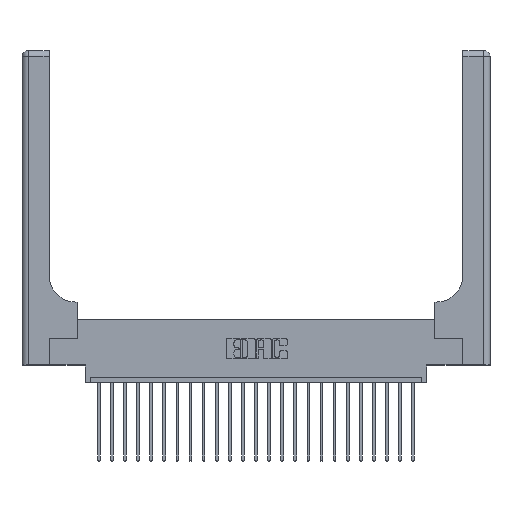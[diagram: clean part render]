
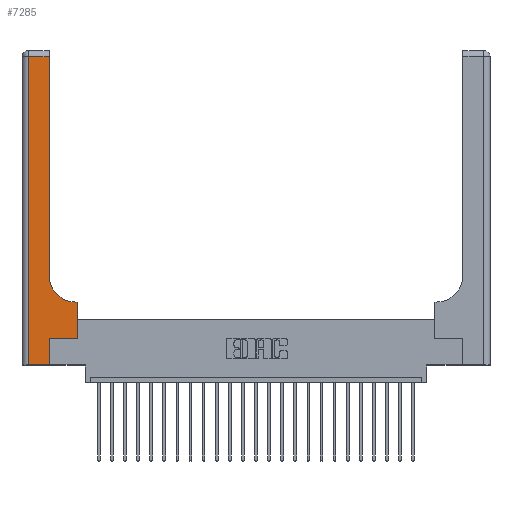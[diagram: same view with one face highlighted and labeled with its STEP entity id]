
A CAD part, top view. The second image highlights one B-rep face of the part: STEP entity #7285.
In plain terms, the highlighted planar face has unit normal (0, 0, 1).
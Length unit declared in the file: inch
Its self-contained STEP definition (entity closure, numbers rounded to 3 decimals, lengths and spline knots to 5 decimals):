
#115 = CARTESIAN_POINT ( 'NONE',  ( 0.528, 0.25, 0.37 ) ) ;
#1245 = CARTESIAN_POINT ( 'NONE',  ( 0., 2.94, 0.37 ) ) ;
#1367 = VERTEX_POINT ( 'NONE', #16172 ) ;
#1421 = CARTESIAN_POINT ( 'NONE',  ( 0.06, 2.94, 0.37 ) ) ;
#1515 = DIRECTION ( 'NONE',  ( -1., 0., 0. ) ) ;
#1929 = CARTESIAN_POINT ( 'NONE',  ( 0.265, 0.25, 0.37 ) ) ;
#2201 = VERTEX_POINT ( 'NONE', #11281 ) ;
#3313 = CARTESIAN_POINT ( 'NONE',  ( 0., 0., 0.37 ) ) ;
#3406 = VECTOR ( 'NONE', #12323, 39.37008 ) ;
#3703 = FACE_OUTER_BOUND ( 'NONE', #9967, .T. ) ;
#3890 = CARTESIAN_POINT ( 'NONE',  ( 0.265, 0., 0.37 ) ) ;
#4806 = EDGE_CURVE ( 'NONE', #6923, #16408, #19016, .T. ) ;
#5321 = CARTESIAN_POINT ( 'NONE',  ( 0., 3., 0.37 ) ) ;
#5400 = DIRECTION ( 'NONE',  ( -1., 0., 0. ) ) ;
#5598 = DIRECTION ( 'NONE',  ( 1., 0., 0. ) ) ;
#6023 = LINE ( 'NONE', #7914, #6333 ) ;
#6162 = ORIENTED_EDGE ( 'NONE', *, *, #16328, .T. ) ;
#6215 = LINE ( 'NONE', #1929, #19160 ) ;
#6298 = CARTESIAN_POINT ( 'NONE',  ( 0.528, 0.6, 0.37 ) ) ;
#6316 = EDGE_CURVE ( 'NONE', #21444, #19864, #19773, .T. ) ;
#6333 = VECTOR ( 'NONE', #20721, 39.37008 ) ;
#6530 = ORIENTED_EDGE ( 'NONE', *, *, #22628, .T. ) ;
#6909 = ORIENTED_EDGE ( 'NONE', *, *, #7799, .T. ) ;
#6923 = VERTEX_POINT ( 'NONE', #11937 ) ;
#7273 = CARTESIAN_POINT ( 'NONE',  ( 0.26, 2.94, 0.37 ) ) ;
#7285 = ADVANCED_FACE ( 'NONE', ( #3703 ), #21324, .F. ) ;
#7539 = VERTEX_POINT ( 'NONE', #6298 ) ;
#7799 = EDGE_CURVE ( 'NONE', #1367, #6923, #17224, .T. ) ;
#7914 = CARTESIAN_POINT ( 'NONE',  ( 0.26, 3., 0.37 ) ) ;
#8052 = CARTESIAN_POINT ( 'NONE',  ( 0.26, 0.85, 0.37 ) ) ;
#8183 = DIRECTION ( 'NONE',  ( -1., 0., 0. ) ) ;
#8191 = VERTEX_POINT ( 'NONE', #8052 ) ;
#8727 = EDGE_CURVE ( 'NONE', #19864, #1367, #14047, .T. ) ;
#8965 = DIRECTION ( 'NONE',  ( 1., 0., 0. ) ) ;
#9324 = VECTOR ( 'NONE', #10646, 39.37008 ) ;
#9737 = EDGE_CURVE ( 'NONE', #7539, #2201, #20332, .T. ) ;
#9857 = CARTESIAN_POINT ( 'NONE',  ( 0.528, 0.25, 0.37 ) ) ;
#9967 = EDGE_LOOP ( 'NONE', ( #6530, #14756, #12165, #6909, #21656, #6162, #17475, #20558, #11203 ) ) ;
#10203 = CIRCLE ( 'NONE', #23147, 0.25 ) ;
#10455 = DIRECTION ( 'NONE',  ( 0., 0., -1. ) ) ;
#10646 = DIRECTION ( 'NONE',  ( 1., 0., 0. ) ) ;
#11150 = CARTESIAN_POINT ( 'NONE',  ( 0.265, 0.25, 0.37 ) ) ;
#11203 = ORIENTED_EDGE ( 'NONE', *, *, #22464, .T. ) ;
#11281 = CARTESIAN_POINT ( 'NONE',  ( 0.51, 0.6, 0.37 ) ) ;
#11849 = DIRECTION ( 'NONE',  ( 0., 1., 0. ) ) ;
#11937 = CARTESIAN_POINT ( 'NONE',  ( 0.265, 0., 0.37 ) ) ;
#12165 = ORIENTED_EDGE ( 'NONE', *, *, #8727, .T. ) ;
#12323 = DIRECTION ( 'NONE',  ( 0., -1., 0. ) ) ;
#14047 = LINE ( 'NONE', #17750, #3406 ) ;
#14324 = CARTESIAN_POINT ( 'NONE',  ( 0.51, 0.85, 0.37 ) ) ;
#14756 = ORIENTED_EDGE ( 'NONE', *, *, #6316, .T. ) ;
#15543 = LINE ( 'NONE', #9857, #20304 ) ;
#15677 = EDGE_CURVE ( 'NONE', #18984, #7539, #15543, .T. ) ;
#16172 = CARTESIAN_POINT ( 'NONE',  ( 0.06, 0., 0.37 ) ) ;
#16216 = VECTOR ( 'NONE', #18117, 39.37008 ) ;
#16328 = EDGE_CURVE ( 'NONE', #16408, #18984, #6215, .T. ) ;
#16408 = VERTEX_POINT ( 'NONE', #11150 ) ;
#17224 = LINE ( 'NONE', #3313, #9324 ) ;
#17475 = ORIENTED_EDGE ( 'NONE', *, *, #15677, .T. ) ;
#17549 = VECTOR ( 'NONE', #8183, 39.37008 ) ;
#17750 = CARTESIAN_POINT ( 'NONE',  ( 0.06, 3., 0.37 ) ) ;
#17965 = DIRECTION ( 'NONE',  ( 0., 0., -1. ) ) ;
#18117 = DIRECTION ( 'NONE',  ( 0., 1., 0. ) ) ;
#18984 = VERTEX_POINT ( 'NONE', #115 ) ;
#19016 = LINE ( 'NONE', #3890, #16216 ) ;
#19160 = VECTOR ( 'NONE', #5598, 39.37008 ) ;
#19624 = CARTESIAN_POINT ( 'NONE',  ( 0.26, 0.6, 0.37 ) ) ;
#19755 = VECTOR ( 'NONE', #5400, 39.37008 ) ;
#19773 = LINE ( 'NONE', #1245, #17549 ) ;
#19864 = VERTEX_POINT ( 'NONE', #1421 ) ;
#20304 = VECTOR ( 'NONE', #11849, 39.37008 ) ;
#20332 = LINE ( 'NONE', #19624, #19755 ) ;
#20498 = AXIS2_PLACEMENT_3D ( 'NONE', #5321, #10455, #1515 ) ;
#20558 = ORIENTED_EDGE ( 'NONE', *, *, #9737, .T. ) ;
#20721 = DIRECTION ( 'NONE',  ( 0., 1., 0. ) ) ;
#21324 = PLANE ( 'NONE',  #20498 ) ;
#21444 = VERTEX_POINT ( 'NONE', #7273 ) ;
#21656 = ORIENTED_EDGE ( 'NONE', *, *, #4806, .T. ) ;
#22464 = EDGE_CURVE ( 'NONE', #2201, #8191, #10203, .T. ) ;
#22628 = EDGE_CURVE ( 'NONE', #8191, #21444, #6023, .T. ) ;
#23147 = AXIS2_PLACEMENT_3D ( 'NONE', #14324, #17965, #8965 ) ;
